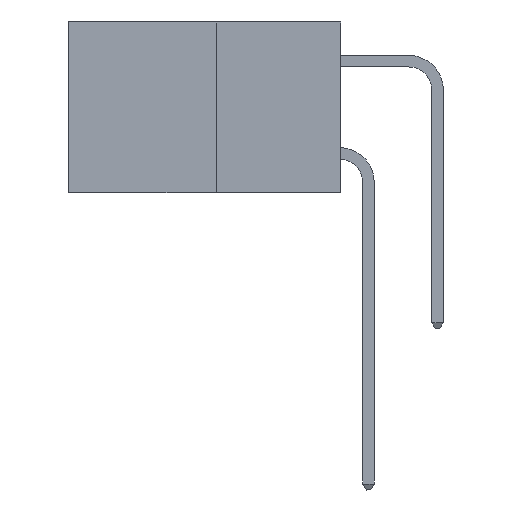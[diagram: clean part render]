
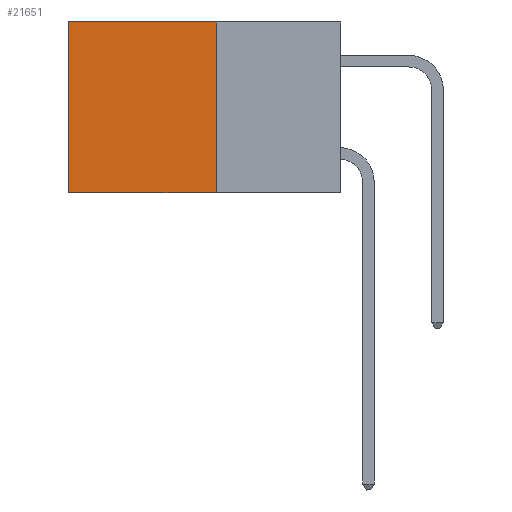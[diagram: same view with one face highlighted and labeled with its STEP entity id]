
A CAD part, left-side view. The second image highlights one B-rep face of the part: STEP entity #21651.
In plain terms, the highlighted planar face has unit normal (-1, 0, 0).
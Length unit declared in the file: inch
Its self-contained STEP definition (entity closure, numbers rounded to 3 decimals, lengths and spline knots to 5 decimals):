
#1196 = DIRECTION ( 'NONE',  ( 1., 0., 0. ) ) ;
#1991 = VECTOR ( 'NONE', #20616, 39.37008 ) ;
#2645 = LINE ( 'NONE', #18498, #1991 ) ;
#2711 = CARTESIAN_POINT ( 'NONE',  ( 0.277, 0.27, 0. ) ) ;
#2785 = EDGE_CURVE ( 'NONE', #8283, #24833, #12218, .T. ) ;
#5370 = CARTESIAN_POINT ( 'NONE',  ( 0.277, 0.27, -0.37 ) ) ;
#5733 = FACE_OUTER_BOUND ( 'NONE', #24408, .T. ) ;
#6465 = ORIENTED_EDGE ( 'NONE', *, *, #10627, .F. ) ;
#7344 = VECTOR ( 'NONE', #25118, 39.37008 ) ;
#7705 = VECTOR ( 'NONE', #24898, 39.37008 ) ;
#8283 = VERTEX_POINT ( 'NONE', #2711 ) ;
#9237 = EDGE_CURVE ( 'NONE', #24833, #26304, #14616, .T. ) ;
#10627 = EDGE_CURVE ( 'NONE', #8283, #25036, #17907, .T. ) ;
#10705 = ORIENTED_EDGE ( 'NONE', *, *, #9237, .T. ) ;
#11655 = CARTESIAN_POINT ( 'NONE',  ( 0.277, 0.27, -0.37 ) ) ;
#12218 = LINE ( 'NONE', #15494, #22178 ) ;
#14237 = CARTESIAN_POINT ( 'NONE',  ( 0.277, 0.59, -0.37 ) ) ;
#14616 = LINE ( 'NONE', #14237, #7705 ) ;
#15311 = EDGE_CURVE ( 'NONE', #25036, #26304, #2645, .T. ) ;
#15494 = CARTESIAN_POINT ( 'NONE',  ( 0.277, 0.27, 0. ) ) ;
#15937 = DIRECTION ( 'NONE',  ( 0., 0., -1. ) ) ;
#16227 = DIRECTION ( 'NONE',  ( 0., 1., 0. ) ) ;
#17464 = CARTESIAN_POINT ( 'NONE',  ( 0.277, 0.59, 0. ) ) ;
#17697 = ORIENTED_EDGE ( 'NONE', *, *, #2785, .T. ) ;
#17907 = LINE ( 'NONE', #23004, #7344 ) ;
#18498 = CARTESIAN_POINT ( 'NONE',  ( 0.277, 0.27, -0.37 ) ) ;
#20616 = DIRECTION ( 'NONE',  ( 0., 1., 0. ) ) ;
#21651 = ADVANCED_FACE ( 'NONE', ( #5733 ), #24364, .F. ) ;
#21990 = ORIENTED_EDGE ( 'NONE', *, *, #15311, .F. ) ;
#22178 = VECTOR ( 'NONE', #16227, 39.37008 ) ;
#23004 = CARTESIAN_POINT ( 'NONE',  ( 0.277, 0.27, -0.37 ) ) ;
#24364 = PLANE ( 'NONE',  #27310 ) ;
#24408 = EDGE_LOOP ( 'NONE', ( #10705, #21990, #6465, #17697 ) ) ;
#24833 = VERTEX_POINT ( 'NONE', #17464 ) ;
#24898 = DIRECTION ( 'NONE',  ( 0., 0., -1. ) ) ;
#25036 = VERTEX_POINT ( 'NONE', #5370 ) ;
#25118 = DIRECTION ( 'NONE',  ( 0., 0., -1. ) ) ;
#26068 = CARTESIAN_POINT ( 'NONE',  ( 0.277, 0.59, -0.37 ) ) ;
#26304 = VERTEX_POINT ( 'NONE', #26068 ) ;
#27310 = AXIS2_PLACEMENT_3D ( 'NONE', #11655, #1196, #15937 ) ;
